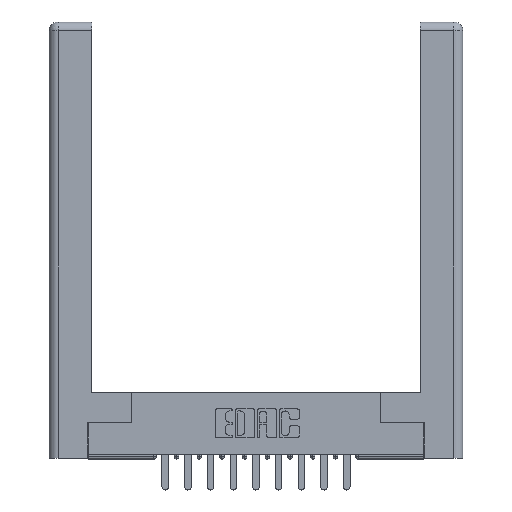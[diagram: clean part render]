
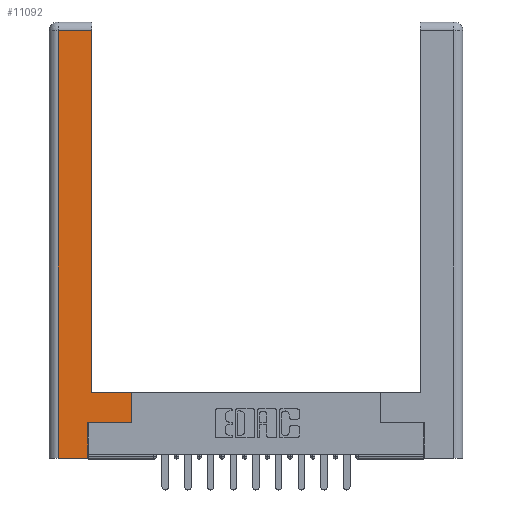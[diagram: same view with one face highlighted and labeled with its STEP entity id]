
A CAD part, top view. The second image highlights one B-rep face of the part: STEP entity #11092.
In plain terms, the highlighted planar face has unit normal (0, 0, 1).
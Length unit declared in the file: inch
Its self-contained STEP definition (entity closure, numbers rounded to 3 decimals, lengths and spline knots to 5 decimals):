
#141 = EDGE_CURVE ( 'NONE', #8169, #2583, #14853, .T. ) ;
#338 = VERTEX_POINT ( 'NONE', #3325 ) ;
#592 = CARTESIAN_POINT ( 'NONE',  ( 0.295, 2.94, 0. ) ) ;
#1464 = ORIENTED_EDGE ( 'NONE', *, *, #2587, .T. ) ;
#1546 = VECTOR ( 'NONE', #12971, 39.37008 ) ;
#1744 = LINE ( 'NONE', #10390, #1546 ) ;
#1823 = EDGE_CURVE ( 'NONE', #13769, #338, #5398, .T. ) ;
#2055 = CARTESIAN_POINT ( 'NONE',  ( 0.0615, 2.94, 0. ) ) ;
#2500 = CARTESIAN_POINT ( 'NONE',  ( 0.565, 0.245, 0. ) ) ;
#2583 = VERTEX_POINT ( 'NONE', #8277 ) ;
#2587 = EDGE_CURVE ( 'NONE', #9884, #13769, #4782, .T. ) ;
#2829 = CARTESIAN_POINT ( 'NONE',  ( 0.295, 3., 0. ) ) ;
#3058 = CARTESIAN_POINT ( 'NONE',  ( 0.295, 0.45, 0. ) ) ;
#3325 = CARTESIAN_POINT ( 'NONE',  ( 0.265, 0., 0. ) ) ;
#3590 = DIRECTION ( 'NONE',  ( 0., 1., 0. ) ) ;
#4049 = VECTOR ( 'NONE', #3590, 39.37008 ) ;
#4698 = DIRECTION ( 'NONE',  ( 1., 0., 0. ) ) ;
#4782 = LINE ( 'NONE', #5685, #15820 ) ;
#4971 = ORIENTED_EDGE ( 'NONE', *, *, #8929, .T. ) ;
#5390 = PLANE ( 'NONE',  #7074 ) ;
#5398 = LINE ( 'NONE', #6033, #10340 ) ;
#5685 = CARTESIAN_POINT ( 'NONE',  ( 0.0615, 0., 0. ) ) ;
#5753 = LINE ( 'NONE', #2500, #8692 ) ;
#5796 = DIRECTION ( 'NONE',  ( 0., 1., 0. ) ) ;
#5847 = LINE ( 'NONE', #16080, #12540 ) ;
#6033 = CARTESIAN_POINT ( 'NONE',  ( 0.265, 0., 0. ) ) ;
#6046 = CARTESIAN_POINT ( 'NONE',  ( 0.0615, 0., 0. ) ) ;
#7074 = AXIS2_PLACEMENT_3D ( 'NONE', #11775, #15467, #12923 ) ;
#7118 = DIRECTION ( 'NONE',  ( 0., -1., 0. ) ) ;
#7539 = VERTEX_POINT ( 'NONE', #592 ) ;
#7626 = CARTESIAN_POINT ( 'NONE',  ( 0.265, 0.245, 0. ) ) ;
#7662 = LINE ( 'NONE', #2829, #10017 ) ;
#7918 = EDGE_CURVE ( 'NONE', #7539, #9884, #1744, .T. ) ;
#8169 = VERTEX_POINT ( 'NONE', #9743 ) ;
#8230 = VECTOR ( 'NONE', #11371, 39.37008 ) ;
#8255 = ORIENTED_EDGE ( 'NONE', *, *, #7918, .T. ) ;
#8277 = CARTESIAN_POINT ( 'NONE',  ( 0.565, 0.45, 0. ) ) ;
#8422 = CARTESIAN_POINT ( 'NONE',  ( 0.565, 0.45, 0. ) ) ;
#8518 = FACE_OUTER_BOUND ( 'NONE', #12129, .T. ) ;
#8692 = VECTOR ( 'NONE', #15863, 39.37008 ) ;
#8929 = EDGE_CURVE ( 'NONE', #16008, #7539, #7662, .T. ) ;
#9488 = EDGE_CURVE ( 'NONE', #338, #10406, #16072, .T. ) ;
#9743 = CARTESIAN_POINT ( 'NONE',  ( 0.565, 0.245, 0. ) ) ;
#9884 = VERTEX_POINT ( 'NONE', #2055 ) ;
#10017 = VECTOR ( 'NONE', #5796, 39.37008 ) ;
#10340 = VECTOR ( 'NONE', #4698, 39.37008 ) ;
#10390 = CARTESIAN_POINT ( 'NONE',  ( 0.0615, 2.94, 0. ) ) ;
#10406 = VERTEX_POINT ( 'NONE', #12370 ) ;
#10610 = EDGE_CURVE ( 'NONE', #10406, #8169, #5753, .T. ) ;
#11092 = ADVANCED_FACE ( 'NONE', ( #8518 ), #5390, .F. ) ;
#11371 = DIRECTION ( 'NONE',  ( 0., 1., 0. ) ) ;
#11775 = CARTESIAN_POINT ( 'NONE',  ( 0., 0., 0. ) ) ;
#11908 = ORIENTED_EDGE ( 'NONE', *, *, #10610, .T. ) ;
#12129 = EDGE_LOOP ( 'NONE', ( #4971, #8255, #1464, #16024, #14834, #11908, #13833, #12964 ) ) ;
#12370 = CARTESIAN_POINT ( 'NONE',  ( 0.265, 0.245, 0. ) ) ;
#12540 = VECTOR ( 'NONE', #14906, 39.37008 ) ;
#12923 = DIRECTION ( 'NONE',  ( -1., 0., 0. ) ) ;
#12964 = ORIENTED_EDGE ( 'NONE', *, *, #13720, .T. ) ;
#12971 = DIRECTION ( 'NONE',  ( -1., 0., 0. ) ) ;
#13720 = EDGE_CURVE ( 'NONE', #2583, #16008, #5847, .T. ) ;
#13769 = VERTEX_POINT ( 'NONE', #6046 ) ;
#13833 = ORIENTED_EDGE ( 'NONE', *, *, #141, .T. ) ;
#14834 = ORIENTED_EDGE ( 'NONE', *, *, #9488, .T. ) ;
#14853 = LINE ( 'NONE', #8422, #4049 ) ;
#14906 = DIRECTION ( 'NONE',  ( -1., 0., 0. ) ) ;
#15467 = DIRECTION ( 'NONE',  ( 0., 0., -1. ) ) ;
#15820 = VECTOR ( 'NONE', #7118, 39.37008 ) ;
#15863 = DIRECTION ( 'NONE',  ( 1., 0., 0. ) ) ;
#16008 = VERTEX_POINT ( 'NONE', #3058 ) ;
#16024 = ORIENTED_EDGE ( 'NONE', *, *, #1823, .T. ) ;
#16072 = LINE ( 'NONE', #7626, #8230 ) ;
#16080 = CARTESIAN_POINT ( 'NONE',  ( 0.295, 0.45, 0. ) ) ;
